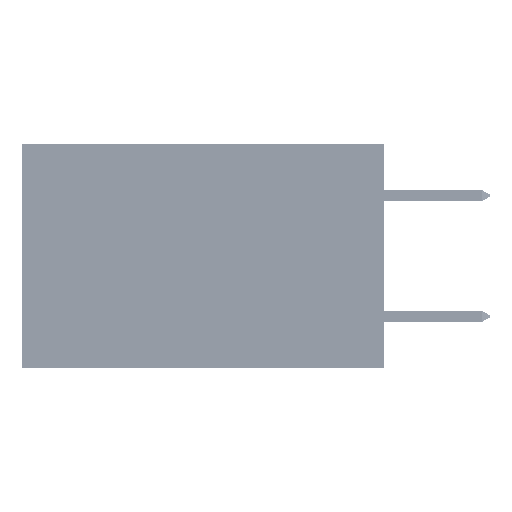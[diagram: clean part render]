
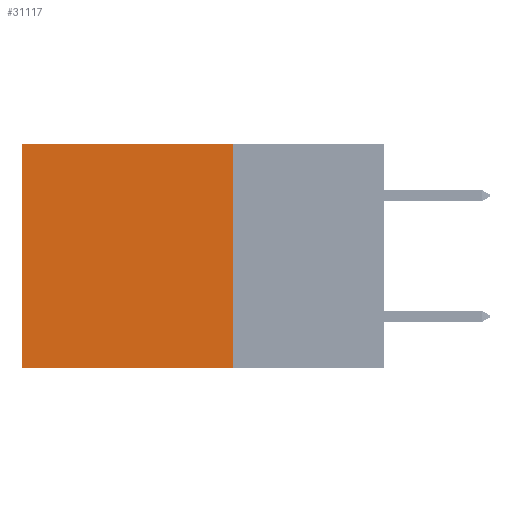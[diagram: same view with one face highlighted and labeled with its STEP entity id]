
A CAD part, left-side view. The second image highlights one B-rep face of the part: STEP entity #31117.
In plain terms, the highlighted planar face has unit normal (-1, 0, 0).
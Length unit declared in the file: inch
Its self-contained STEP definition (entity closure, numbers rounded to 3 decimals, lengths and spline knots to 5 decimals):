
#1560 = LINE ( 'NONE', #16284, #32598 ) ;
#2302 = CARTESIAN_POINT ( 'NONE',  ( 0.2875, 0.25, 0. ) ) ;
#2503 = CARTESIAN_POINT ( 'NONE',  ( 0.2875, 0.25, 0. ) ) ;
#4125 = DIRECTION ( 'NONE',  ( 0., 1., 0. ) ) ;
#6187 = EDGE_CURVE ( 'NONE', #33198, #49229, #34761, .T. ) ;
#8485 = CARTESIAN_POINT ( 'NONE',  ( 0.2875, 0.25, -0.37 ) ) ;
#9761 = LINE ( 'NONE', #35804, #51442 ) ;
#13401 = EDGE_CURVE ( 'NONE', #49229, #36688, #51152, .T. ) ;
#13459 = FACE_OUTER_BOUND ( 'NONE', #40658, .T. ) ;
#13669 = CARTESIAN_POINT ( 'NONE',  ( 0.2875, 0.6, 0. ) ) ;
#15836 = DIRECTION ( 'NONE',  ( 0., 0., -1. ) ) ;
#16284 = CARTESIAN_POINT ( 'NONE',  ( 0.2875, 0.25, 0. ) ) ;
#17476 = DIRECTION ( 'NONE',  ( 0., 0., -1. ) ) ;
#17731 = VECTOR ( 'NONE', #36642, 39.37008 ) ;
#22987 = EDGE_CURVE ( 'NONE', #48775, #36688, #9761, .T. ) ;
#30800 = DIRECTION ( 'NONE',  ( 0., 0., -1. ) ) ;
#31117 = ADVANCED_FACE ( 'NONE', ( #13459 ), #37476, .F. ) ;
#32598 = VECTOR ( 'NONE', #4125, 39.37008 ) ;
#33108 = CARTESIAN_POINT ( 'NONE',  ( 0.2875, 0.25, -0.37 ) ) ;
#33198 = VERTEX_POINT ( 'NONE', #2302 ) ;
#33418 = CARTESIAN_POINT ( 'NONE',  ( 0.2875, 0.25, 0. ) ) ;
#34761 = LINE ( 'NONE', #2503, #45531 ) ;
#35804 = CARTESIAN_POINT ( 'NONE',  ( 0.2875, 0.6, 0. ) ) ;
#36642 = DIRECTION ( 'NONE',  ( 0., 1., 0. ) ) ;
#36688 = VERTEX_POINT ( 'NONE', #48064 ) ;
#37476 = PLANE ( 'NONE',  #41738 ) ;
#37483 = ORIENTED_EDGE ( 'NONE', *, *, #6187, .F. ) ;
#40658 = EDGE_LOOP ( 'NONE', ( #41150, #41048, #37483, #52320 ) ) ;
#41048 = ORIENTED_EDGE ( 'NONE', *, *, #13401, .F. ) ;
#41150 = ORIENTED_EDGE ( 'NONE', *, *, #22987, .T. ) ;
#41519 = DIRECTION ( 'NONE',  ( 1., 0., 0. ) ) ;
#41738 = AXIS2_PLACEMENT_3D ( 'NONE', #33418, #41519, #17476 ) ;
#45531 = VECTOR ( 'NONE', #30800, 39.37008 ) ;
#47179 = EDGE_CURVE ( 'NONE', #33198, #48775, #1560, .T. ) ;
#48064 = CARTESIAN_POINT ( 'NONE',  ( 0.2875, 0.6, -0.37 ) ) ;
#48775 = VERTEX_POINT ( 'NONE', #13669 ) ;
#49229 = VERTEX_POINT ( 'NONE', #33108 ) ;
#51152 = LINE ( 'NONE', #8485, #17731 ) ;
#51442 = VECTOR ( 'NONE', #15836, 39.37008 ) ;
#52320 = ORIENTED_EDGE ( 'NONE', *, *, #47179, .T. ) ;
